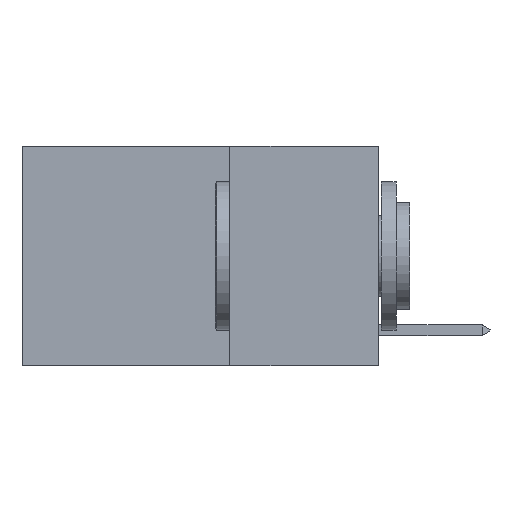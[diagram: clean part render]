
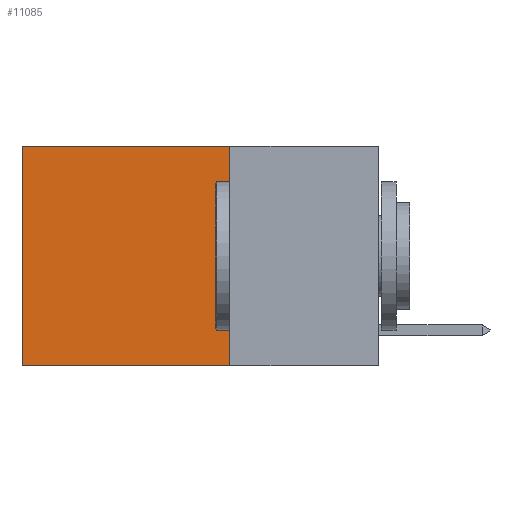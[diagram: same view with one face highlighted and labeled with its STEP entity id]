
A CAD part, left-side view. The second image highlights one B-rep face of the part: STEP entity #11085.
In plain terms, the highlighted planar face has unit normal (-1, 0, 0).
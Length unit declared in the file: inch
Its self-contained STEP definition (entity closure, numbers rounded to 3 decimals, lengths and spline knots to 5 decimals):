
#39 = VERTEX_POINT ( 'NONE', #9679 ) ;
#98 = VECTOR ( 'NONE', #395, 39.37008 ) ;
#144 = FACE_OUTER_BOUND ( 'NONE', #1931, .T. ) ;
#395 = DIRECTION ( 'NONE',  ( 0., 1., 0. ) ) ;
#804 = CARTESIAN_POINT ( 'NONE',  ( 0.2625, 0.6, -0.37 ) ) ;
#1440 = VERTEX_POINT ( 'NONE', #2316 ) ;
#1931 = EDGE_LOOP ( 'NONE', ( #15390, #11291, #13395, #6208 ) ) ;
#2104 = CARTESIAN_POINT ( 'NONE',  ( 0.2625, 0.25, 0. ) ) ;
#2316 = CARTESIAN_POINT ( 'NONE',  ( 0.2625, 0.25, 0. ) ) ;
#2482 = CARTESIAN_POINT ( 'NONE',  ( 0.2625, 0.6, 0. ) ) ;
#2601 = EDGE_CURVE ( 'NONE', #6043, #9556, #5019, .T. ) ;
#3093 = EDGE_CURVE ( 'NONE', #1440, #39, #6036, .T. ) ;
#3755 = AXIS2_PLACEMENT_3D ( 'NONE', #12672, #4935, #14877 ) ;
#3971 = CARTESIAN_POINT ( 'NONE',  ( 0.2625, 0.25, -0.37 ) ) ;
#4192 = VECTOR ( 'NONE', #14048, 39.37008 ) ;
#4778 = EDGE_CURVE ( 'NONE', #1440, #6043, #15731, .T. ) ;
#4935 = DIRECTION ( 'NONE',  ( 1., 0., 0. ) ) ;
#5019 = LINE ( 'NONE', #2482, #4192 ) ;
#5952 = DIRECTION ( 'NONE',  ( 0., 0., -1. ) ) ;
#6036 = LINE ( 'NONE', #9955, #13069 ) ;
#6043 = VERTEX_POINT ( 'NONE', #10271 ) ;
#6208 = ORIENTED_EDGE ( 'NONE', *, *, #4778, .T. ) ;
#7057 = DIRECTION ( 'NONE',  ( 0., 1., 0. ) ) ;
#7238 = VECTOR ( 'NONE', #7057, 39.37008 ) ;
#7908 = EDGE_CURVE ( 'NONE', #39, #9556, #9159, .T. ) ;
#9159 = LINE ( 'NONE', #3971, #98 ) ;
#9556 = VERTEX_POINT ( 'NONE', #804 ) ;
#9679 = CARTESIAN_POINT ( 'NONE',  ( 0.2625, 0.25, -0.37 ) ) ;
#9955 = CARTESIAN_POINT ( 'NONE',  ( 0.2625, 0.25, 0. ) ) ;
#10271 = CARTESIAN_POINT ( 'NONE',  ( 0.2625, 0.6, 0. ) ) ;
#11085 = ADVANCED_FACE ( 'NONE', ( #144 ), #11141, .F. ) ;
#11141 = PLANE ( 'NONE',  #3755 ) ;
#11291 = ORIENTED_EDGE ( 'NONE', *, *, #7908, .F. ) ;
#12672 = CARTESIAN_POINT ( 'NONE',  ( 0.2625, 0.25, 0. ) ) ;
#13069 = VECTOR ( 'NONE', #5952, 39.37008 ) ;
#13395 = ORIENTED_EDGE ( 'NONE', *, *, #3093, .F. ) ;
#14048 = DIRECTION ( 'NONE',  ( 0., 0., -1. ) ) ;
#14877 = DIRECTION ( 'NONE',  ( 0., 0., -1. ) ) ;
#15390 = ORIENTED_EDGE ( 'NONE', *, *, #2601, .T. ) ;
#15731 = LINE ( 'NONE', #2104, #7238 ) ;
